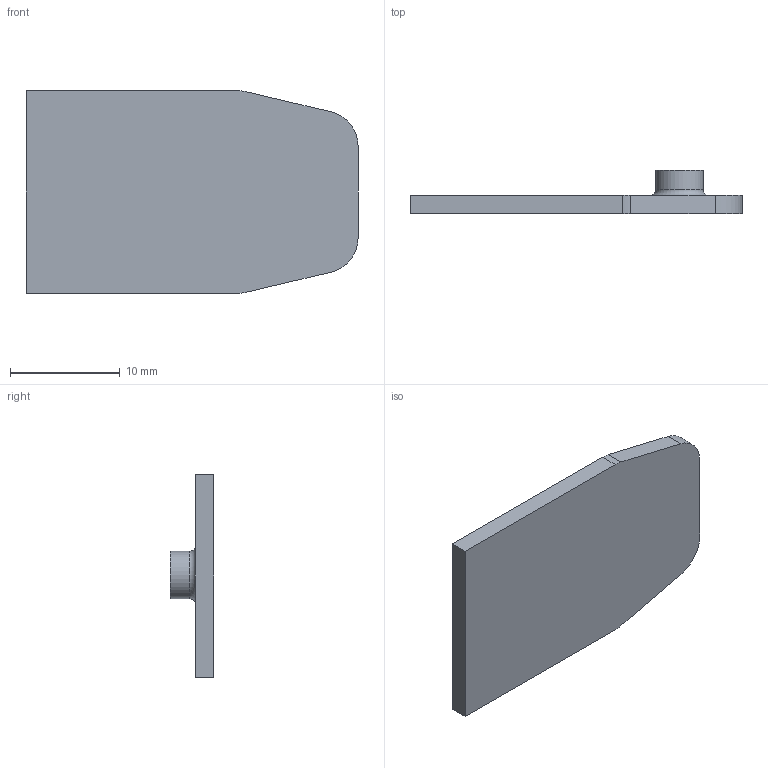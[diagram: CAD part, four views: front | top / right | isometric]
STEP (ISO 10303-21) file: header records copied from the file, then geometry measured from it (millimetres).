
FILE_DESCRIPTION(/* description */ (''),/* implementation_level */ '2;1');
FILE_NAME(/* name */ 'Menendez Mag Locking Tab V1.1.stp',/* time_stamp */ '2019-06-27T23:09:43-05:00',/* author */ ('johne'),/* organization */ (''),/* preprocessor_version */ 'ST-DEVELOPER v16.13',/* originating_system */ 'Autodesk Inventor 2018',/* authorisation */ '');
FILE_SCHEMA (('AUTOMOTIVE_DESIGN { 1 0 10303 214 3 1 1 }'));
Length unit declared in the file: inch
Products named in the file (1): Menendez Mag Follower V1.11
Bounding box: 30.3 x 3.94 x 18.47 mm (x, y, z)
Volume: 910.5 mm3; surface area: 1240.8 mm2
Topology: 1 solids, 1 shells, 15 faces, 35 edges, 23 vertices
Faces by surface type: plane 9, cylinder 5, torus 1
Full cylindrical faces by diameter (mm): 4.318 x1
Entity records: 463 total; most frequent: DIRECTION 76, CARTESIAN_POINT 72, ORIENTED_EDGE 66, EDGE_CURVE 33, AXIS2_PLACEMENT_3D 27, VERTEX_POINT 23, LINE 22, VECTOR 22
